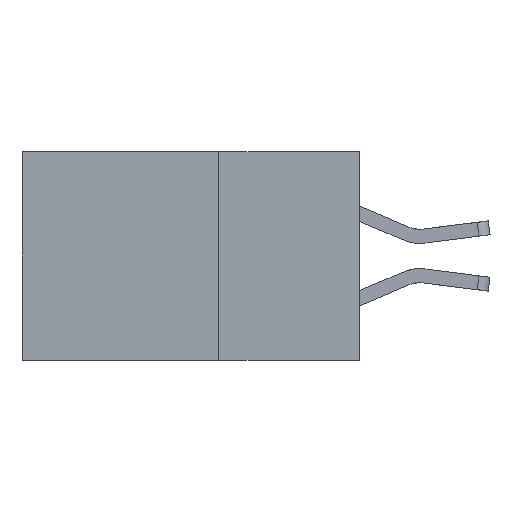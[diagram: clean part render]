
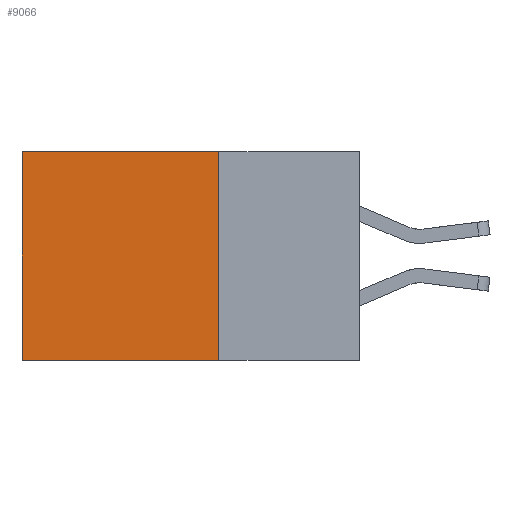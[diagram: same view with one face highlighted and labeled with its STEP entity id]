
A CAD part, left-side view. The second image highlights one B-rep face of the part: STEP entity #9066.
In plain terms, the highlighted planar face has unit normal (-1, 0, 0).
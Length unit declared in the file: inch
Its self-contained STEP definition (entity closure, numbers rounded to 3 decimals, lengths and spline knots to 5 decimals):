
#275 = EDGE_CURVE ( 'NONE', #10772, #9719, #9713, .T. ) ;
#363 = CARTESIAN_POINT ( 'NONE',  ( 0.2875, 0.6, 0. ) ) ;
#883 = CARTESIAN_POINT ( 'NONE',  ( 0.2875, 0.25, -0.37 ) ) ;
#907 = PLANE ( 'NONE',  #2488 ) ;
#1004 = CARTESIAN_POINT ( 'NONE',  ( 0.2875, 0.25, -0.37 ) ) ;
#1606 = DIRECTION ( 'NONE',  ( 0., 0., -1. ) ) ;
#2488 = AXIS2_PLACEMENT_3D ( 'NONE', #3509, #6897, #2692 ) ;
#2502 = VECTOR ( 'NONE', #7274, 39.37008 ) ;
#2521 = CARTESIAN_POINT ( 'NONE',  ( 0.2875, 0.6, -0.37 ) ) ;
#2692 = DIRECTION ( 'NONE',  ( 0., 0., -1. ) ) ;
#2840 = VECTOR ( 'NONE', #9505, 39.37008 ) ;
#3154 = ORIENTED_EDGE ( 'NONE', *, *, #9884, .F. ) ;
#3221 = CARTESIAN_POINT ( 'NONE',  ( 0.2875, 0.6, 0. ) ) ;
#3509 = CARTESIAN_POINT ( 'NONE',  ( 0.2875, 0.25, 0. ) ) ;
#4156 = VERTEX_POINT ( 'NONE', #883 ) ;
#4436 = EDGE_LOOP ( 'NONE', ( #6390, #3154, #9184, #9962 ) ) ;
#5673 = VERTEX_POINT ( 'NONE', #10235 ) ;
#5940 = CARTESIAN_POINT ( 'NONE',  ( 0.2875, 0.25, 0. ) ) ;
#6117 = CARTESIAN_POINT ( 'NONE',  ( 0.2875, 0.25, 0. ) ) ;
#6390 = ORIENTED_EDGE ( 'NONE', *, *, #275, .T. ) ;
#6897 = DIRECTION ( 'NONE',  ( 1., 0., 0. ) ) ;
#6954 = DIRECTION ( 'NONE',  ( 0., 1., 0. ) ) ;
#7012 = FACE_OUTER_BOUND ( 'NONE', #4436, .T. ) ;
#7274 = DIRECTION ( 'NONE',  ( 0., 1., 0. ) ) ;
#7717 = EDGE_CURVE ( 'NONE', #5673, #10772, #9332, .T. ) ;
#8610 = LINE ( 'NONE', #1004, #2502 ) ;
#9066 = ADVANCED_FACE ( 'NONE', ( #7012 ), #907, .F. ) ;
#9080 = EDGE_CURVE ( 'NONE', #5673, #4156, #10333, .T. ) ;
#9184 = ORIENTED_EDGE ( 'NONE', *, *, #9080, .F. ) ;
#9332 = LINE ( 'NONE', #5940, #9761 ) ;
#9505 = DIRECTION ( 'NONE',  ( 0., 0., -1. ) ) ;
#9713 = LINE ( 'NONE', #3221, #9901 ) ;
#9719 = VERTEX_POINT ( 'NONE', #2521 ) ;
#9761 = VECTOR ( 'NONE', #6954, 39.37008 ) ;
#9884 = EDGE_CURVE ( 'NONE', #4156, #9719, #8610, .T. ) ;
#9901 = VECTOR ( 'NONE', #1606, 39.37008 ) ;
#9962 = ORIENTED_EDGE ( 'NONE', *, *, #7717, .T. ) ;
#10235 = CARTESIAN_POINT ( 'NONE',  ( 0.2875, 0.25, 0. ) ) ;
#10333 = LINE ( 'NONE', #6117, #2840 ) ;
#10772 = VERTEX_POINT ( 'NONE', #363 ) ;
